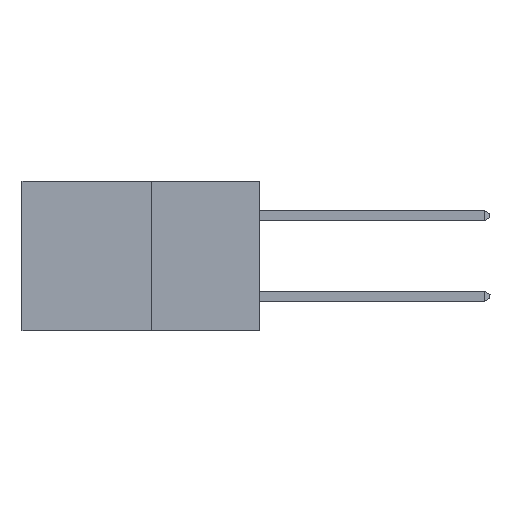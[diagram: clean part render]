
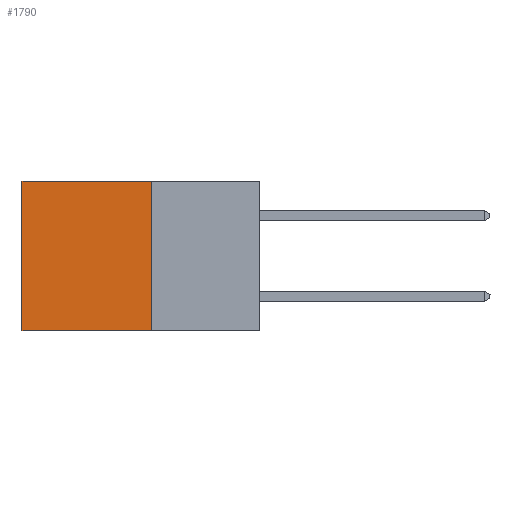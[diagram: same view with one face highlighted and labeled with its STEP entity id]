
A CAD part, left-side view. The second image highlights one B-rep face of the part: STEP entity #1790.
In plain terms, the highlighted planar face has unit normal (-1, 0, 0).
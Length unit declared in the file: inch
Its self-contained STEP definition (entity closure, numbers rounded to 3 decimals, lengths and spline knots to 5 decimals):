
#303 = EDGE_CURVE ( 'NONE', #6156, #5697, #6221, .T. ) ;
#331 = ORIENTED_EDGE ( 'NONE', *, *, #1017, .F. ) ;
#600 = ORIENTED_EDGE ( 'NONE', *, *, #2987, .F. ) ;
#1017 = EDGE_CURVE ( 'NONE', #6156, #6203, #5808, .T. ) ;
#1267 = CARTESIAN_POINT ( 'NONE',  ( 0.277, 0.27, 0. ) ) ;
#1500 = EDGE_LOOP ( 'NONE', ( #3386, #600, #331, #5346 ) ) ;
#1570 = VECTOR ( 'NONE', #1830, 39.37008 ) ;
#1714 = AXIS2_PLACEMENT_3D ( 'NONE', #4781, #5475, #1795 ) ;
#1790 = ADVANCED_FACE ( 'NONE', ( #7707 ), #5204, .F. ) ;
#1795 = DIRECTION ( 'NONE',  ( 0., 0., -1. ) ) ;
#1830 = DIRECTION ( 'NONE',  ( 0., 1., 0. ) ) ;
#2176 = VECTOR ( 'NONE', #7000, 39.37008 ) ;
#2251 = VERTEX_POINT ( 'NONE', #6075 ) ;
#2987 = EDGE_CURVE ( 'NONE', #6203, #2251, #3274, .T. ) ;
#3088 = VECTOR ( 'NONE', #4116, 39.37008 ) ;
#3274 = LINE ( 'NONE', #7753, #2176 ) ;
#3386 = ORIENTED_EDGE ( 'NONE', *, *, #4354, .T. ) ;
#4054 = DIRECTION ( 'NONE',  ( 0., 0., -1. ) ) ;
#4116 = DIRECTION ( 'NONE',  ( 0., 0., -1. ) ) ;
#4354 = EDGE_CURVE ( 'NONE', #5697, #2251, #6168, .T. ) ;
#4668 = CARTESIAN_POINT ( 'NONE',  ( 0.277, 0.27, -0.37 ) ) ;
#4781 = CARTESIAN_POINT ( 'NONE',  ( 0.277, 0.27, -0.37 ) ) ;
#5204 = PLANE ( 'NONE',  #1714 ) ;
#5223 = CARTESIAN_POINT ( 'NONE',  ( 0.277, 0.27, -0.37 ) ) ;
#5346 = ORIENTED_EDGE ( 'NONE', *, *, #303, .T. ) ;
#5444 = CARTESIAN_POINT ( 'NONE',  ( 0.277, 0.59, 0. ) ) ;
#5475 = DIRECTION ( 'NONE',  ( 1., 0., 0. ) ) ;
#5634 = VECTOR ( 'NONE', #4054, 39.37008 ) ;
#5697 = VERTEX_POINT ( 'NONE', #5444 ) ;
#5808 = LINE ( 'NONE', #5223, #5634 ) ;
#6075 = CARTESIAN_POINT ( 'NONE',  ( 0.277, 0.59, -0.37 ) ) ;
#6156 = VERTEX_POINT ( 'NONE', #1267 ) ;
#6168 = LINE ( 'NONE', #7408, #3088 ) ;
#6203 = VERTEX_POINT ( 'NONE', #4668 ) ;
#6221 = LINE ( 'NONE', #7443, #1570 ) ;
#7000 = DIRECTION ( 'NONE',  ( 0., 1., 0. ) ) ;
#7408 = CARTESIAN_POINT ( 'NONE',  ( 0.277, 0.59, -0.37 ) ) ;
#7443 = CARTESIAN_POINT ( 'NONE',  ( 0.277, 0.27, 0. ) ) ;
#7707 = FACE_OUTER_BOUND ( 'NONE', #1500, .T. ) ;
#7753 = CARTESIAN_POINT ( 'NONE',  ( 0.277, 0.27, -0.37 ) ) ;
